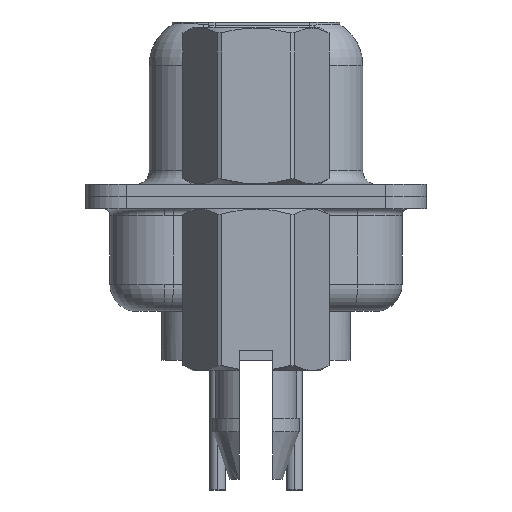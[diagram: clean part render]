
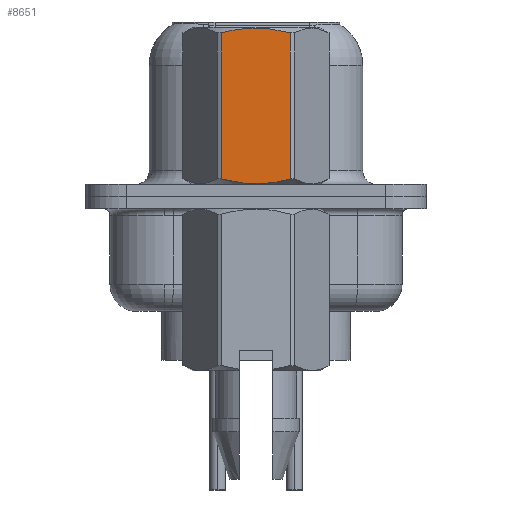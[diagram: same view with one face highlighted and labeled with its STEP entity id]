
A CAD part, left-side view. The second image highlights one B-rep face of the part: STEP entity #8651.
In plain terms, the highlighted planar face has unit normal (-1, 0, 0).
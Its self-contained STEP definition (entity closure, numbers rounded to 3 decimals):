
#1052 = FACE_OUTER_BOUND ( 'NONE', #20708, .T. ) ;
#1106 = CARTESIAN_POINT ( 'NONE',  ( -2.381, 1.273, 3.792 ) ) ;
#1703 = VECTOR ( 'NONE', #10407, 1000. ) ;
#3567 = CARTESIAN_POINT ( 'NONE',  ( -2.381, 0.428, 6.215 ) ) ;
#5232 = CARTESIAN_POINT ( 'NONE',  ( -2.381, -1.066, 6.104 ) ) ;
#5350 = CARTESIAN_POINT ( 'NONE',  ( -2.381, -1.273, 0.652 ) ) ;
#5377 = CARTESIAN_POINT ( 'NONE',  ( -2.381, 0.853, 6.151 ) ) ;
#5503 = ORIENTED_EDGE ( 'NONE', *, *, #10653, .T. ) ;
#5670 = CARTESIAN_POINT ( 'NONE',  ( -2.381, -0.215, 6.232 ) ) ;
#6494 = EDGE_CURVE ( 'NONE', #11436, #22214, #20536, .T. ) ;
#6746 = VERTEX_POINT ( 'NONE', #25275 ) ;
#7102 = VECTOR ( 'NONE', #11888, 1000. ) ;
#7337 = CARTESIAN_POINT ( 'NONE',  ( -2.381, -0.432, 6.215 ) ) ;
#7619 = CARTESIAN_POINT ( 'NONE',  ( -2.381, 1.273, 6.048 ) ) ;
#7781 = DIRECTION ( 'NONE',  ( 0., -1., 0. ) ) ;
#8257 = CARTESIAN_POINT ( 'NONE',  ( -2.381, -0.858, 0.55 ) ) ;
#8651 = ADVANCED_FACE ( 'NONE', ( #1052 ), #26640, .T. ) ;
#8897 = CARTESIAN_POINT ( 'NONE',  ( -2.381, -1.273, 6.048 ) ) ;
#9609 = EDGE_CURVE ( 'NONE', #11470, #6746, #21279, .T. ) ;
#10407 = DIRECTION ( 'NONE',  ( 0., 0., 1. ) ) ;
#10653 = EDGE_CURVE ( 'NONE', #6746, #11436, #14370, .T. ) ;
#11436 = VERTEX_POINT ( 'NONE', #26330 ) ;
#11470 = VERTEX_POINT ( 'NONE', #18365 ) ;
#11527 = CARTESIAN_POINT ( 'NONE',  ( -2.381, -0.858, 6.15 ) ) ;
#11888 = DIRECTION ( 'NONE',  ( 0., 0., -1. ) ) ;
#11971 = CARTESIAN_POINT ( 'NONE',  ( -2.381, 1.375, -3.75 ) ) ;
#12125 = CARTESIAN_POINT ( 'NONE',  ( -2.381, 1.273, 0.652 ) ) ;
#13889 = CARTESIAN_POINT ( 'NONE',  ( -2.381, 0.428, 0.485 ) ) ;
#14030 = CARTESIAN_POINT ( 'NONE',  ( -2.381, -1.066, 0.596 ) ) ;
#14079 = DIRECTION ( 'NONE',  ( -1., 0., 0. ) ) ;
#14370 = B_SPLINE_CURVE_WITH_KNOTS ( 'NONE', 3,
 ( #8897, #5232, #11527, #7337, #5670, #26902, #3567, #5377, #22397, #7619 ),
 .UNSPECIFIED., .F., .F.,
 ( 4, 2, 2, 2, 4 ),
 ( 0.001, 0.002, 0.002, 0.003, 0.004 ),
 .UNSPECIFIED. ) ;
#16577 = EDGE_CURVE ( 'NONE', #22214, #11470, #22496, .T. ) ;
#16741 = ORIENTED_EDGE ( 'NONE', *, *, #16577, .T. ) ;
#17149 = ORIENTED_EDGE ( 'NONE', *, *, #6494, .T. ) ;
#18365 = CARTESIAN_POINT ( 'NONE',  ( -2.381, -1.273, 0.652 ) ) ;
#19638 = AXIS2_PLACEMENT_3D ( 'NONE', #11971, #14079, #7781 ) ;
#20019 = CARTESIAN_POINT ( 'NONE',  ( -2.381, 0.215, 0.468 ) ) ;
#20536 = LINE ( 'NONE', #1106, #7102 ) ;
#20708 = EDGE_LOOP ( 'NONE', ( #16741, #25638, #5503, #17149 ) ) ;
#21279 = LINE ( 'NONE', #23233, #1703 ) ;
#22214 = VERTEX_POINT ( 'NONE', #12125 ) ;
#22397 = CARTESIAN_POINT ( 'NONE',  ( -2.381, 1.065, 6.104 ) ) ;
#22496 = B_SPLINE_CURVE_WITH_KNOTS ( 'NONE', 3,
 ( #26595, #27260, #24494, #13889, #20019, #24201, #27392, #8257, #14030, #5350 ),
 .UNSPECIFIED., .F., .F.,
 ( 4, 2, 2, 2, 4 ),
 ( 0.003, 0.003, 0.004, 0.004, 0.005 ),
 .UNSPECIFIED. ) ;
#23233 = CARTESIAN_POINT ( 'NONE',  ( -2.381, -1.273, 3.792 ) ) ;
#24201 = CARTESIAN_POINT ( 'NONE',  ( -2.381, -0.215, 0.468 ) ) ;
#24494 = CARTESIAN_POINT ( 'NONE',  ( -2.381, 0.853, 0.549 ) ) ;
#25275 = CARTESIAN_POINT ( 'NONE',  ( -2.381, -1.273, 6.048 ) ) ;
#25638 = ORIENTED_EDGE ( 'NONE', *, *, #9609, .T. ) ;
#26330 = CARTESIAN_POINT ( 'NONE',  ( -2.381, 1.273, 6.048 ) ) ;
#26595 = CARTESIAN_POINT ( 'NONE',  ( -2.381, 1.273, 0.652 ) ) ;
#26640 = PLANE ( 'NONE',  #19638 ) ;
#26902 = CARTESIAN_POINT ( 'NONE',  ( -2.381, 0.215, 6.232 ) ) ;
#27260 = CARTESIAN_POINT ( 'NONE',  ( -2.381, 1.065, 0.596 ) ) ;
#27392 = CARTESIAN_POINT ( 'NONE',  ( -2.381, -0.432, 0.485 ) ) ;
